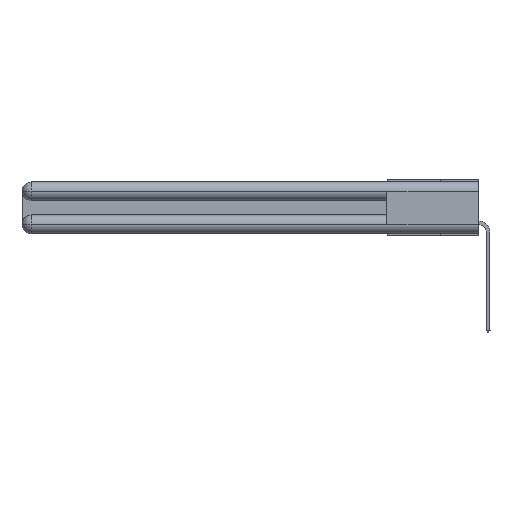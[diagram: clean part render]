
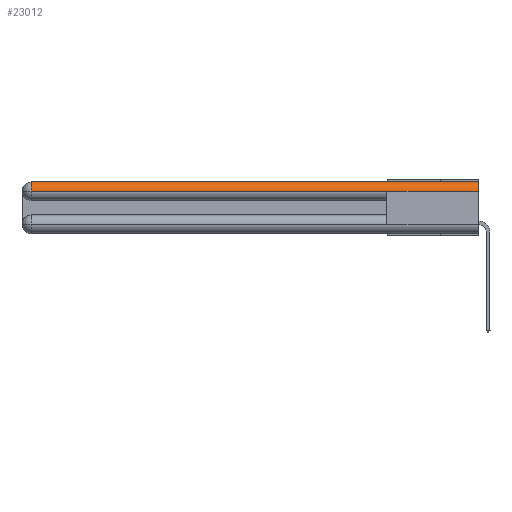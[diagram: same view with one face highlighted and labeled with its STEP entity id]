
A CAD part, left-side view. The second image highlights one B-rep face of the part: STEP entity #23012.
In plain terms, the highlighted cylindrical face has radius 1.562 mm (diameter 3.124 mm), a partial arc.
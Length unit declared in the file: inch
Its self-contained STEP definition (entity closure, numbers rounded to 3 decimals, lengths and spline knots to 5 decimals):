
#1129 = DIRECTION ( 'NONE',  ( 0., -1., 0. ) ) ;
#1163 = CARTESIAN_POINT ( 'NONE',  ( 0.0615, 2.94, 0. ) ) ;
#1997 = DIRECTION ( 'NONE',  ( 0., -1., 0. ) ) ;
#2089 = DIRECTION ( 'NONE',  ( 0., -1., 0. ) ) ;
#3484 = LINE ( 'NONE', #21102, #23382 ) ;
#4497 = DIRECTION ( 'NONE',  ( 0., -1., 0. ) ) ;
#5146 = ORIENTED_EDGE ( 'NONE', *, *, #14533, .T. ) ;
#5337 = LINE ( 'NONE', #20718, #13342 ) ;
#5390 = VERTEX_POINT ( 'NONE', #7303 ) ;
#5863 = AXIS2_PLACEMENT_3D ( 'NONE', #15681, #1997, #19912 ) ;
#7303 = CARTESIAN_POINT ( 'NONE',  ( 0., 0.6, -0.0615 ) ) ;
#7652 = VECTOR ( 'NONE', #4497, 39.37008 ) ;
#8284 = LINE ( 'NONE', #20858, #7652 ) ;
#8345 = VERTEX_POINT ( 'NONE', #1163 ) ;
#9696 = VERTEX_POINT ( 'NONE', #26174 ) ;
#9934 = EDGE_CURVE ( 'NONE', #8345, #9696, #8284, .T. ) ;
#10017 = CIRCLE ( 'NONE', #5863, 0.0615 ) ;
#11327 = CARTESIAN_POINT ( 'NONE',  ( 0.0615, 0., -0.0615 ) ) ;
#11525 = EDGE_CURVE ( 'NONE', #9696, #16195, #10017, .T. ) ;
#12086 = ORIENTED_EDGE ( 'NONE', *, *, #9934, .F. ) ;
#13254 = CARTESIAN_POINT ( 'NONE',  ( 0.0615, 2.94, -0.0615 ) ) ;
#13342 = VECTOR ( 'NONE', #2089, 39.37008 ) ;
#14082 = EDGE_CURVE ( 'NONE', #16195, #5390, #3484, .T. ) ;
#14533 = EDGE_CURVE ( 'NONE', #18675, #5390, #5337, .T. ) ;
#15681 = CARTESIAN_POINT ( 'NONE',  ( 0.0615, 0., -0.0615 ) ) ;
#16024 = AXIS2_PLACEMENT_3D ( 'NONE', #11327, #23990, #19767 ) ;
#16195 = VERTEX_POINT ( 'NONE', #24667 ) ;
#18016 = ORIENTED_EDGE ( 'NONE', *, *, #11525, .F. ) ;
#18333 = CIRCLE ( 'NONE', #22834, 0.0615 ) ;
#18415 = FACE_OUTER_BOUND ( 'NONE', #21723, .T. ) ;
#18602 = CARTESIAN_POINT ( 'NONE',  ( 0., 2.94, -0.0615 ) ) ;
#18675 = VERTEX_POINT ( 'NONE', #18602 ) ;
#19183 = DIRECTION ( 'NONE',  ( 0., 1., 0. ) ) ;
#19254 = EDGE_CURVE ( 'NONE', #8345, #18675, #18333, .T. ) ;
#19767 = DIRECTION ( 'NONE',  ( 0., 0., 1. ) ) ;
#19912 = DIRECTION ( 'NONE',  ( 1., 0., 0. ) ) ;
#20718 = CARTESIAN_POINT ( 'NONE',  ( 0., 3., -0.0615 ) ) ;
#20858 = CARTESIAN_POINT ( 'NONE',  ( 0.0615, 0., 0. ) ) ;
#21019 = CYLINDRICAL_SURFACE ( 'NONE', #16024, 0.0615 ) ;
#21102 = CARTESIAN_POINT ( 'NONE',  ( 0., 3., -0.0615 ) ) ;
#21723 = EDGE_LOOP ( 'NONE', ( #12086, #24050, #5146, #25104, #18016 ) ) ;
#22834 = AXIS2_PLACEMENT_3D ( 'NONE', #13254, #1129, #25574 ) ;
#23012 = ADVANCED_FACE ( 'NONE', ( #18415 ), #21019, .T. ) ;
#23382 = VECTOR ( 'NONE', #19183, 39.37008 ) ;
#23990 = DIRECTION ( 'NONE',  ( 0., 1., 0. ) ) ;
#24050 = ORIENTED_EDGE ( 'NONE', *, *, #19254, .T. ) ;
#24667 = CARTESIAN_POINT ( 'NONE',  ( 0., 0., -0.0615 ) ) ;
#25104 = ORIENTED_EDGE ( 'NONE', *, *, #14082, .F. ) ;
#25574 = DIRECTION ( 'NONE',  ( 0., 0., 1. ) ) ;
#26174 = CARTESIAN_POINT ( 'NONE',  ( 0.0615, 0., 0. ) ) ;
